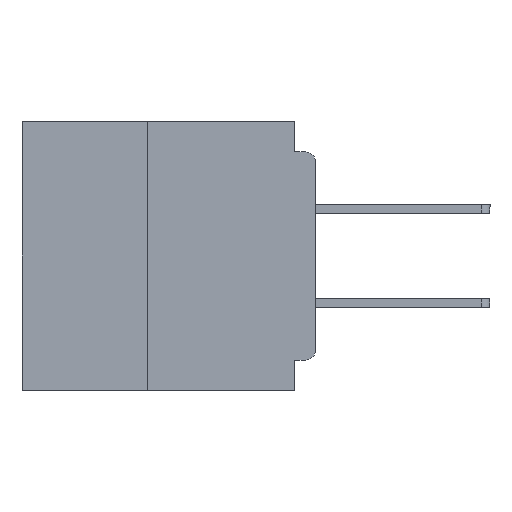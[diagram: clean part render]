
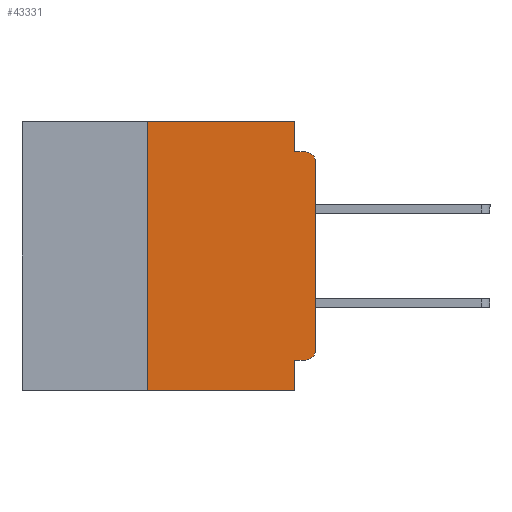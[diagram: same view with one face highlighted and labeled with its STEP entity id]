
A CAD part, left-side view. The second image highlights one B-rep face of the part: STEP entity #43331.
In plain terms, the highlighted planar face has unit normal (-1, 0, 0).
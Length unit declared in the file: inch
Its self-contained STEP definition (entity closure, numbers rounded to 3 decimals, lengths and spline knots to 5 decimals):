
#671 = CARTESIAN_POINT ( 'NONE',  ( 0., 0.25, -0.4 ) ) ;
#1269 = CARTESIAN_POINT ( 'NONE',  ( 0., 0.437, 0. ) ) ;
#1513 = CARTESIAN_POINT ( 'NONE',  ( 0., 0.437, 0. ) ) ;
#3049 = DIRECTION ( 'NONE',  ( 0., 0., -1. ) ) ;
#3087 = CARTESIAN_POINT ( 'NONE',  ( 0., 0., -0.355 ) ) ;
#3520 = ORIENTED_EDGE ( 'NONE', *, *, #19987, .T. ) ;
#3777 = ORIENTED_EDGE ( 'NONE', *, *, #7704, .T. ) ;
#4385 = DIRECTION ( 'NONE',  ( 0., 0., 1. ) ) ;
#4752 = CARTESIAN_POINT ( 'NONE',  ( 0., 0.031, -0.4 ) ) ;
#5010 = LINE ( 'NONE', #32187, #31384 ) ;
#5055 = VERTEX_POINT ( 'NONE', #34484 ) ;
#5681 = ORIENTED_EDGE ( 'NONE', *, *, #29327, .F. ) ;
#5987 = CARTESIAN_POINT ( 'NONE',  ( 0., 0., -0.045 ) ) ;
#6843 = VECTOR ( 'NONE', #37338, 39.37008 ) ;
#7058 = CIRCLE ( 'NONE', #15318, 0.015 ) ;
#7137 = EDGE_CURVE ( 'NONE', #7752, #29070, #28762, .T. ) ;
#7206 = EDGE_CURVE ( 'NONE', #29070, #29122, #17479, .T. ) ;
#7223 = VECTOR ( 'NONE', #19043, 39.37008 ) ;
#7704 = EDGE_CURVE ( 'NONE', #43207, #5055, #5010, .T. ) ;
#7752 = VERTEX_POINT ( 'NONE', #15258 ) ;
#8052 = CARTESIAN_POINT ( 'NONE',  ( 0., 0.015, -0.06 ) ) ;
#9511 = VECTOR ( 'NONE', #15197, 39.37008 ) ;
#10532 = ORIENTED_EDGE ( 'NONE', *, *, #17589, .F. ) ;
#11548 = DIRECTION ( 'NONE',  ( 0., 0., -1. ) ) ;
#11653 = DIRECTION ( 'NONE',  ( 0., -1., 0. ) ) ;
#11703 = EDGE_LOOP ( 'NONE', ( #23528, #3520, #35511, #34585, #32204, #15558, #3777, #10532, #5681, #28023 ) ) ;
#11751 = DIRECTION ( 'NONE',  ( 1., 0., 0. ) ) ;
#13835 = VERTEX_POINT ( 'NONE', #32329 ) ;
#14666 = EDGE_CURVE ( 'NONE', #35584, #13835, #14678, .T. ) ;
#14678 = LINE ( 'NONE', #14862, #21612 ) ;
#14862 = CARTESIAN_POINT ( 'NONE',  ( 0., 0., 0. ) ) ;
#15197 = DIRECTION ( 'NONE',  ( 0., 0., -1. ) ) ;
#15258 = CARTESIAN_POINT ( 'NONE',  ( 0., 0.25, 0. ) ) ;
#15318 = AXIS2_PLACEMENT_3D ( 'NONE', #8052, #32088, #11548 ) ;
#15558 = ORIENTED_EDGE ( 'NONE', *, *, #43753, .F. ) ;
#16969 = CARTESIAN_POINT ( 'NONE',  ( 0., 0.015, -0.045 ) ) ;
#17252 = CARTESIAN_POINT ( 'NONE',  ( 0., 0.25, -0.4 ) ) ;
#17479 = LINE ( 'NONE', #26115, #7223 ) ;
#17589 = EDGE_CURVE ( 'NONE', #31131, #5055, #18652, .T. ) ;
#18652 = LINE ( 'NONE', #4752, #9511 ) ;
#18964 = EDGE_CURVE ( 'NONE', #29122, #20784, #33527, .T. ) ;
#19043 = DIRECTION ( 'NONE',  ( 0., 0., -1. ) ) ;
#19633 = VECTOR ( 'NONE', #32530, 39.37008 ) ;
#19688 = EDGE_CURVE ( 'NONE', #39691, #35584, #28083, .T. ) ;
#19871 = DIRECTION ( 'NONE',  ( 0., -1., 0. ) ) ;
#19987 = EDGE_CURVE ( 'NONE', #13835, #20784, #7058, .T. ) ;
#20748 = AXIS2_PLACEMENT_3D ( 'NONE', #44135, #23709, #3049 ) ;
#20784 = VERTEX_POINT ( 'NONE', #16969 ) ;
#21612 = VECTOR ( 'NONE', #4385, 39.37008 ) ;
#22563 = CARTESIAN_POINT ( 'NONE',  ( 0., 0.031, -0.045 ) ) ;
#23528 = ORIENTED_EDGE ( 'NONE', *, *, #14666, .T. ) ;
#23709 = DIRECTION ( 'NONE',  ( -1., 0., 0. ) ) ;
#24432 = VECTOR ( 'NONE', #19871, 39.37008 ) ;
#26115 = CARTESIAN_POINT ( 'NONE',  ( 0., 0.031, 0. ) ) ;
#27316 = LINE ( 'NONE', #17252, #34245 ) ;
#27607 = DIRECTION ( 'NONE',  ( 0., 0., 1. ) ) ;
#27615 = CARTESIAN_POINT ( 'NONE',  ( 0., 0.015, -0.355 ) ) ;
#28023 = ORIENTED_EDGE ( 'NONE', *, *, #19688, .T. ) ;
#28083 = CIRCLE ( 'NONE', #20748, 0.015 ) ;
#28762 = LINE ( 'NONE', #1513, #19633 ) ;
#29070 = VERTEX_POINT ( 'NONE', #32609 ) ;
#29122 = VERTEX_POINT ( 'NONE', #22563 ) ;
#29327 = EDGE_CURVE ( 'NONE', #39691, #31131, #35318, .T. ) ;
#31131 = VERTEX_POINT ( 'NONE', #43574 ) ;
#31384 = VECTOR ( 'NONE', #11653, 39.37008 ) ;
#32088 = DIRECTION ( 'NONE',  ( -1., 0., 0. ) ) ;
#32187 = CARTESIAN_POINT ( 'NONE',  ( 0., 0.437, -0.4 ) ) ;
#32204 = ORIENTED_EDGE ( 'NONE', *, *, #7137, .F. ) ;
#32295 = PLANE ( 'NONE',  #42674 ) ;
#32329 = CARTESIAN_POINT ( 'NONE',  ( 0., 0., -0.06 ) ) ;
#32530 = DIRECTION ( 'NONE',  ( 0., -1., 0. ) ) ;
#32609 = CARTESIAN_POINT ( 'NONE',  ( 0., 0.031, 0. ) ) ;
#33527 = LINE ( 'NONE', #5987, #24432 ) ;
#34245 = VECTOR ( 'NONE', #27607, 39.37008 ) ;
#34484 = CARTESIAN_POINT ( 'NONE',  ( 0., 0.031, -0.4 ) ) ;
#34585 = ORIENTED_EDGE ( 'NONE', *, *, #7206, .F. ) ;
#35318 = LINE ( 'NONE', #3087, #6843 ) ;
#35511 = ORIENTED_EDGE ( 'NONE', *, *, #18964, .F. ) ;
#35584 = VERTEX_POINT ( 'NONE', #36021 ) ;
#35695 = DIRECTION ( 'NONE',  ( 0., 0., -1. ) ) ;
#36021 = CARTESIAN_POINT ( 'NONE',  ( 0., 0., -0.34 ) ) ;
#37338 = DIRECTION ( 'NONE',  ( 0., 1., 0. ) ) ;
#39691 = VERTEX_POINT ( 'NONE', #27615 ) ;
#40572 = FACE_OUTER_BOUND ( 'NONE', #11703, .T. ) ;
#42674 = AXIS2_PLACEMENT_3D ( 'NONE', #1269, #11751, #35695 ) ;
#43207 = VERTEX_POINT ( 'NONE', #671 ) ;
#43331 = ADVANCED_FACE ( 'NONE', ( #40572 ), #32295, .F. ) ;
#43574 = CARTESIAN_POINT ( 'NONE',  ( 0., 0.031, -0.355 ) ) ;
#43753 = EDGE_CURVE ( 'NONE', #43207, #7752, #27316, .T. ) ;
#44135 = CARTESIAN_POINT ( 'NONE',  ( 0., 0.015, -0.34 ) ) ;
